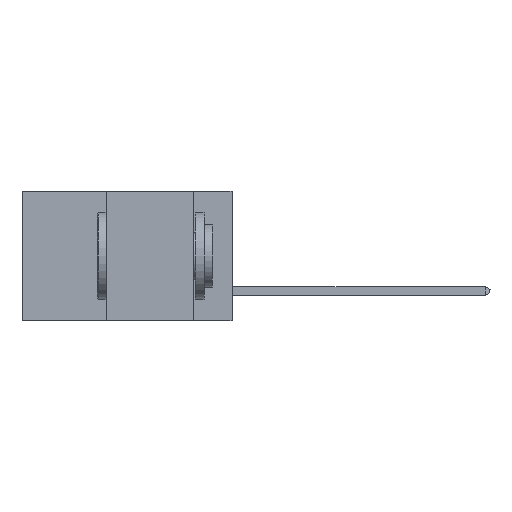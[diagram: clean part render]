
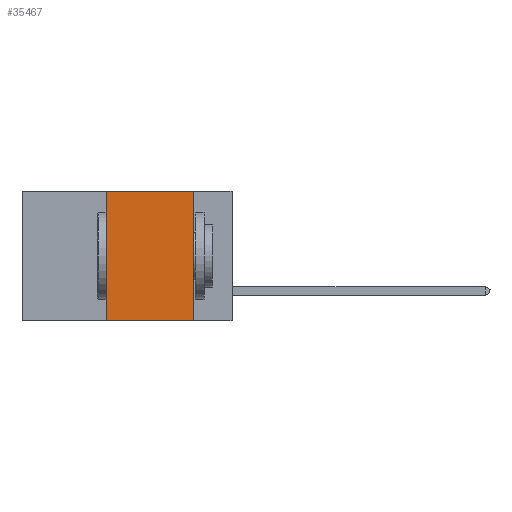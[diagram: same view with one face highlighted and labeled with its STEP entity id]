
A CAD part, left-side view. The second image highlights one B-rep face of the part: STEP entity #35467.
In plain terms, the highlighted planar face has unit normal (-1, 0, 0).
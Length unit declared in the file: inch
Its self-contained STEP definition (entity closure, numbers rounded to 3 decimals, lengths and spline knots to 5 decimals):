
#243 = ORIENTED_EDGE ( 'NONE', *, *, #22004, .F. ) ;
#1767 = DIRECTION ( 'NONE',  ( 0., -1., 0. ) ) ;
#2679 = CARTESIAN_POINT ( 'NONE',  ( 0., 0.11, 0. ) ) ;
#3880 = VECTOR ( 'NONE', #12222, 39.37008 ) ;
#3982 = VERTEX_POINT ( 'NONE', #2679 ) ;
#4508 = ORIENTED_EDGE ( 'NONE', *, *, #32785, .T. ) ;
#4721 = CARTESIAN_POINT ( 'NONE',  ( 0., 0.6, 0. ) ) ;
#5015 = LINE ( 'NONE', #12034, #20783 ) ;
#5389 = LINE ( 'NONE', #18903, #21640 ) ;
#7435 = DIRECTION ( 'NONE',  ( 1., 0., 0. ) ) ;
#7937 = ORIENTED_EDGE ( 'NONE', *, *, #22429, .F. ) ;
#10270 = PLANE ( 'NONE',  #22855 ) ;
#10404 = DIRECTION ( 'NONE',  ( 0., 0., -1. ) ) ;
#10416 = VERTEX_POINT ( 'NONE', #15312 ) ;
#10648 = DIRECTION ( 'NONE',  ( 0., 0., -1. ) ) ;
#12034 = CARTESIAN_POINT ( 'NONE',  ( 0., 0.6, 0. ) ) ;
#12222 = DIRECTION ( 'NONE',  ( 0., 0., 1. ) ) ;
#14515 = CARTESIAN_POINT ( 'NONE',  ( 0., 0.11, -0.37 ) ) ;
#15128 = VERTEX_POINT ( 'NONE', #26024 ) ;
#15312 = CARTESIAN_POINT ( 'NONE',  ( 0., 0.36, 0. ) ) ;
#17400 = DIRECTION ( 'NONE',  ( 0., -1., 0. ) ) ;
#18451 = EDGE_LOOP ( 'NONE', ( #7937, #243, #27993, #4508 ) ) ;
#18628 = VECTOR ( 'NONE', #10648, 39.37008 ) ;
#18903 = CARTESIAN_POINT ( 'NONE',  ( 0., 0.6, -0.37 ) ) ;
#19363 = FACE_OUTER_BOUND ( 'NONE', #18451, .T. ) ;
#19851 = VERTEX_POINT ( 'NONE', #14515 ) ;
#20783 = VECTOR ( 'NONE', #17400, 39.37008 ) ;
#21640 = VECTOR ( 'NONE', #1767, 39.37008 ) ;
#22004 = EDGE_CURVE ( 'NONE', #10416, #3982, #5015, .T. ) ;
#22429 = EDGE_CURVE ( 'NONE', #3982, #19851, #26018, .T. ) ;
#22855 = AXIS2_PLACEMENT_3D ( 'NONE', #4721, #7435, #10404 ) ;
#26018 = LINE ( 'NONE', #35436, #18628 ) ;
#26024 = CARTESIAN_POINT ( 'NONE',  ( 0., 0.36, -0.37 ) ) ;
#26328 = LINE ( 'NONE', #31584, #3880 ) ;
#27993 = ORIENTED_EDGE ( 'NONE', *, *, #28119, .F. ) ;
#28119 = EDGE_CURVE ( 'NONE', #15128, #10416, #26328, .T. ) ;
#31584 = CARTESIAN_POINT ( 'NONE',  ( 0., 0.36, 0. ) ) ;
#32785 = EDGE_CURVE ( 'NONE', #15128, #19851, #5389, .T. ) ;
#35436 = CARTESIAN_POINT ( 'NONE',  ( 0., 0.11, 0. ) ) ;
#35467 = ADVANCED_FACE ( 'NONE', ( #19363 ), #10270, .F. ) ;
